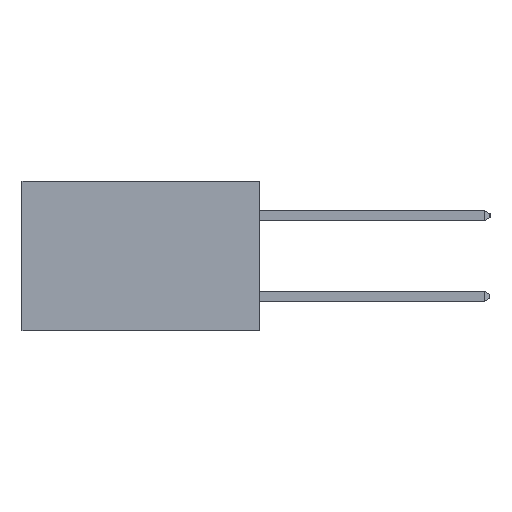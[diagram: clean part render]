
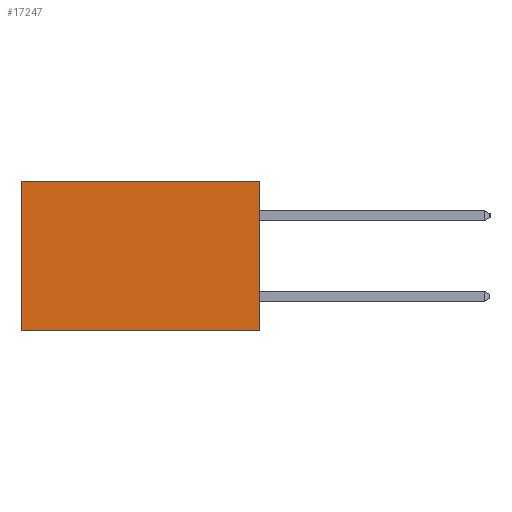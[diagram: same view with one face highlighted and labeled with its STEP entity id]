
A CAD part, left-side view. The second image highlights one B-rep face of the part: STEP entity #17247.
In plain terms, the highlighted planar face has unit normal (-1, 0, 0).
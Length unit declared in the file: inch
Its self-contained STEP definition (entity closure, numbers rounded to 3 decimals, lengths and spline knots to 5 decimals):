
#731 = DIRECTION ( 'NONE',  ( 0., 0., -1. ) ) ;
#2264 = ORIENTED_EDGE ( 'NONE', *, *, #10312, .T. ) ;
#2703 = CARTESIAN_POINT ( 'NONE',  ( 0.277, 0.59, 0. ) ) ;
#3418 = VECTOR ( 'NONE', #22655, 39.37008 ) ;
#3445 = CARTESIAN_POINT ( 'NONE',  ( 0.277, 0., -0.37 ) ) ;
#3746 = CARTESIAN_POINT ( 'NONE',  ( 0.277, 0.59, -0.37 ) ) ;
#3992 = VECTOR ( 'NONE', #15770, 39.37008 ) ;
#4184 = EDGE_LOOP ( 'NONE', ( #16591, #19725, #21774, #2264 ) ) ;
#7328 = VERTEX_POINT ( 'NONE', #9360 ) ;
#8242 = VERTEX_POINT ( 'NONE', #2703 ) ;
#9360 = CARTESIAN_POINT ( 'NONE',  ( 0.277, 0., -0.37 ) ) ;
#9500 = DIRECTION ( 'NONE',  ( 0., 0., -1. ) ) ;
#10312 = EDGE_CURVE ( 'NONE', #13086, #8242, #28294, .T. ) ;
#11814 = CARTESIAN_POINT ( 'NONE',  ( 0.277, 0., 0. ) ) ;
#13086 = VERTEX_POINT ( 'NONE', #14800 ) ;
#14602 = EDGE_CURVE ( 'NONE', #7328, #17657, #21878, .T. ) ;
#14800 = CARTESIAN_POINT ( 'NONE',  ( 0.277, 0., 0. ) ) ;
#14961 = VECTOR ( 'NONE', #19025, 39.37008 ) ;
#15770 = DIRECTION ( 'NONE',  ( 0., 0., -1. ) ) ;
#16550 = AXIS2_PLACEMENT_3D ( 'NONE', #21449, #23786, #9500 ) ;
#16591 = ORIENTED_EDGE ( 'NONE', *, *, #19594, .T. ) ;
#17247 = ADVANCED_FACE ( 'NONE', ( #25102 ), #19057, .F. ) ;
#17657 = VERTEX_POINT ( 'NONE', #25126 ) ;
#17854 = VECTOR ( 'NONE', #731, 39.37008 ) ;
#19025 = DIRECTION ( 'NONE',  ( 0., 1., 0. ) ) ;
#19057 = PLANE ( 'NONE',  #16550 ) ;
#19594 = EDGE_CURVE ( 'NONE', #8242, #17657, #29338, .T. ) ;
#19725 = ORIENTED_EDGE ( 'NONE', *, *, #14602, .F. ) ;
#21449 = CARTESIAN_POINT ( 'NONE',  ( 0.277, 0., -0.37 ) ) ;
#21774 = ORIENTED_EDGE ( 'NONE', *, *, #22377, .F. ) ;
#21878 = LINE ( 'NONE', #3445, #3418 ) ;
#22377 = EDGE_CURVE ( 'NONE', #13086, #7328, #29589, .T. ) ;
#22655 = DIRECTION ( 'NONE',  ( 0., 1., 0. ) ) ;
#23786 = DIRECTION ( 'NONE',  ( 1., 0., 0. ) ) ;
#25102 = FACE_OUTER_BOUND ( 'NONE', #4184, .T. ) ;
#25126 = CARTESIAN_POINT ( 'NONE',  ( 0.277, 0.59, -0.37 ) ) ;
#26966 = CARTESIAN_POINT ( 'NONE',  ( 0.277, 0., -0.37 ) ) ;
#28294 = LINE ( 'NONE', #11814, #14961 ) ;
#29338 = LINE ( 'NONE', #3746, #3992 ) ;
#29589 = LINE ( 'NONE', #26966, #17854 ) ;
